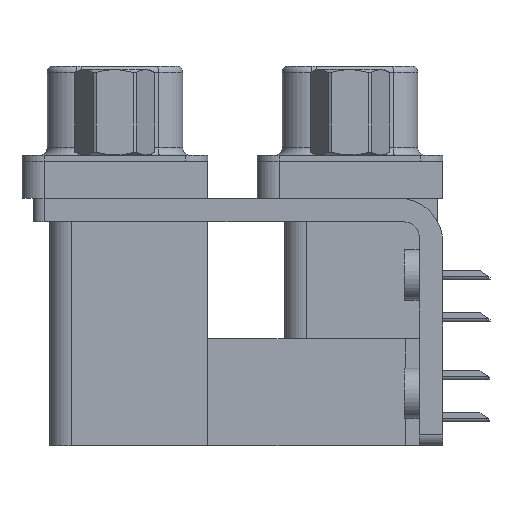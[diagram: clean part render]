
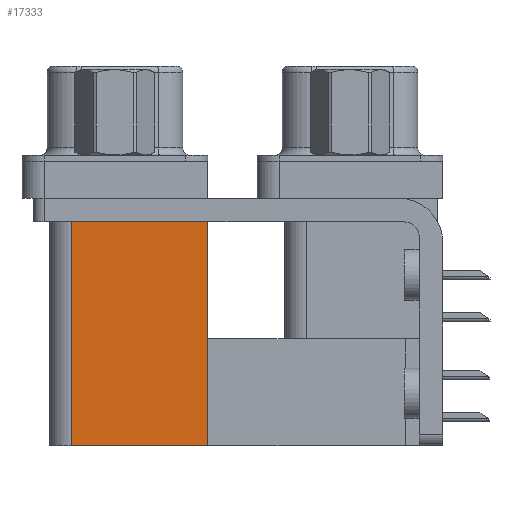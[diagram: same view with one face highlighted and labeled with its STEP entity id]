
A CAD part, left-side view. The second image highlights one B-rep face of the part: STEP entity #17333.
In plain terms, the highlighted planar face has unit normal (-1, 0, 0).
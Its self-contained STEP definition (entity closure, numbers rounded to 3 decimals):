
#1230 = VERTEX_POINT ( 'NONE', #35941 ) ;
#2988 = EDGE_CURVE ( 'NONE', #35824, #1230, #10706, .T. ) ;
#3145 = DIRECTION ( 'NONE',  ( 0., 0., -1. ) ) ;
#3646 = LINE ( 'NONE', #24552, #30282 ) ;
#4127 = VECTOR ( 'NONE', #24650, 1000. ) ;
#4225 = ORIENTED_EDGE ( 'NONE', *, *, #20352, .T. ) ;
#6009 = VECTOR ( 'NONE', #31813, 1000. ) ;
#6473 = DIRECTION ( 'NONE',  ( 1., 0., 0. ) ) ;
#7290 = EDGE_CURVE ( 'NONE', #17739, #29973, #3646, .T. ) ;
#9306 = ORIENTED_EDGE ( 'NONE', *, *, #7290, .F. ) ;
#9713 = LINE ( 'NONE', #16378, #22296 ) ;
#10309 = CARTESIAN_POINT ( 'NONE',  ( 3.765, 9.6, -19.2 ) ) ;
#10706 = LINE ( 'NONE', #10309, #6009 ) ;
#15203 = CARTESIAN_POINT ( 'NONE',  ( 3.765, 18.8, -2.5 ) ) ;
#16078 = CARTESIAN_POINT ( 'NONE',  ( 3.765, 9.6, -2.5 ) ) ;
#16378 = CARTESIAN_POINT ( 'NONE',  ( 3.765, 9.6, -19.2 ) ) ;
#16846 = ORIENTED_EDGE ( 'NONE', *, *, #2988, .T. ) ;
#17333 = ADVANCED_FACE ( 'NONE', ( #29719 ), #27175, .F. ) ;
#17739 = VERTEX_POINT ( 'NONE', #32727 ) ;
#20352 = EDGE_CURVE ( 'NONE', #1230, #29973, #24844, .T. ) ;
#22296 = VECTOR ( 'NONE', #33574, 1000. ) ;
#24552 = CARTESIAN_POINT ( 'NONE',  ( 3.765, 18.8, -19.2 ) ) ;
#24573 = AXIS2_PLACEMENT_3D ( 'NONE', #26599, #6473, #3145 ) ;
#24650 = DIRECTION ( 'NONE',  ( 0., 1., 0. ) ) ;
#24844 = LINE ( 'NONE', #16078, #4127 ) ;
#25607 = EDGE_LOOP ( 'NONE', ( #4225, #9306, #27448, #16846 ) ) ;
#26599 = CARTESIAN_POINT ( 'NONE',  ( 3.765, 9.6, -19.2 ) ) ;
#27175 = PLANE ( 'NONE',  #24573 ) ;
#27448 = ORIENTED_EDGE ( 'NONE', *, *, #38623, .F. ) ;
#29719 = FACE_OUTER_BOUND ( 'NONE', #25607, .T. ) ;
#29973 = VERTEX_POINT ( 'NONE', #15203 ) ;
#30282 = VECTOR ( 'NONE', #33567, 1000. ) ;
#31719 = CARTESIAN_POINT ( 'NONE',  ( 3.765, 9.6, -19.2 ) ) ;
#31813 = DIRECTION ( 'NONE',  ( 0., 0., 1. ) ) ;
#32727 = CARTESIAN_POINT ( 'NONE',  ( 3.765, 18.8, -19.2 ) ) ;
#33567 = DIRECTION ( 'NONE',  ( 0., 0., 1. ) ) ;
#33574 = DIRECTION ( 'NONE',  ( 0., 1., 0. ) ) ;
#35824 = VERTEX_POINT ( 'NONE', #31719 ) ;
#35941 = CARTESIAN_POINT ( 'NONE',  ( 3.765, 9.6, -2.5 ) ) ;
#38623 = EDGE_CURVE ( 'NONE', #35824, #17739, #9713, .T. ) ;
